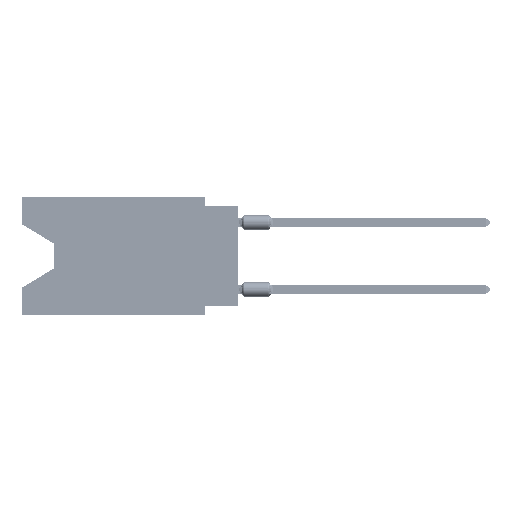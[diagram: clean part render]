
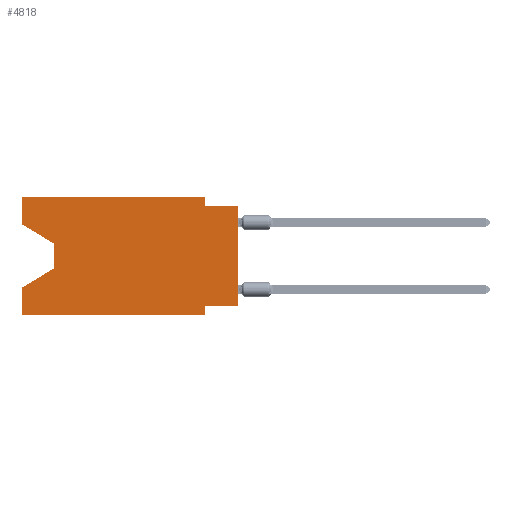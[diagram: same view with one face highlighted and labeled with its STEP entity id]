
A CAD part, left-side view. The second image highlights one B-rep face of the part: STEP entity #4818.
In plain terms, the highlighted planar face has unit normal (-1, 0, 0).
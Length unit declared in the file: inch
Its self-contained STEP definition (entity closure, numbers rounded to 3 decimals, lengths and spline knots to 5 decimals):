
#1222 = DIRECTION ( 'NONE',  ( 1., 0., 0. ) ) ;
#3884 = VERTEX_POINT ( 'NONE', #79119 ) ;
#4818 = ADVANCED_FACE ( 'NONE', ( #48601 ), #41045, .F. ) ;
#5077 = CARTESIAN_POINT ( 'NONE',  ( 0., 0.1, -0.35 ) ) ;
#6990 = VECTOR ( 'NONE', #43015, 39.37008 ) ;
#8329 = DIRECTION ( 'NONE',  ( 0., 0., -1. ) ) ;
#11922 = VERTEX_POINT ( 'NONE', #38605 ) ;
#16854 = DIRECTION ( 'NONE',  ( 0., 0., -1. ) ) ;
#16881 = VERTEX_POINT ( 'NONE', #51182 ) ;
#18978 = ORIENTED_EDGE ( 'NONE', *, *, #21117, .T. ) ;
#19656 = VERTEX_POINT ( 'NONE', #95528 ) ;
#19881 = VERTEX_POINT ( 'NONE', #33614 ) ;
#19899 = EDGE_CURVE ( 'NONE', #19881, #81661, #68547, .T. ) ;
#21117 = EDGE_CURVE ( 'NONE', #92996, #19881, #44362, .T. ) ;
#22657 = CARTESIAN_POINT ( 'NONE',  ( 0., 0.1, -0.35 ) ) ;
#23414 = CARTESIAN_POINT ( 'NONE',  ( 0., 0.645, -0.35 ) ) ;
#23574 = CARTESIAN_POINT ( 'NONE',  ( 0., 0.645, 0. ) ) ;
#24090 = LINE ( 'NONE', #23574, #85095 ) ;
#24146 = CARTESIAN_POINT ( 'NONE',  ( 0., 0.1, -0.325 ) ) ;
#24910 = CARTESIAN_POINT ( 'NONE',  ( 0., 0.645, 0. ) ) ;
#29621 = VECTOR ( 'NONE', #73208, 39.37008 ) ;
#30368 = VERTEX_POINT ( 'NONE', #24146 ) ;
#30608 = CARTESIAN_POINT ( 'NONE',  ( 0., 0.1, -0.025 ) ) ;
#31564 = ORIENTED_EDGE ( 'NONE', *, *, #97087, .F. ) ;
#31740 = DIRECTION ( 'NONE',  ( 0., 0., 1. ) ) ;
#33614 = CARTESIAN_POINT ( 'NONE',  ( 0., 0.55, -0.212 ) ) ;
#35190 = DIRECTION ( 'NONE',  ( 0., 0.855, -0.519 ) ) ;
#36057 = EDGE_CURVE ( 'NONE', #19656, #81661, #96804, .T. ) ;
#37345 = AXIS2_PLACEMENT_3D ( 'NONE', #24910, #1222, #16854 ) ;
#38605 = CARTESIAN_POINT ( 'NONE',  ( 0., 0., -0.325 ) ) ;
#40043 = DIRECTION ( 'NONE',  ( 0., -1., 0. ) ) ;
#40207 = DIRECTION ( 'NONE',  ( 0., -1., 0. ) ) ;
#40370 = VECTOR ( 'NONE', #35190, 39.37008 ) ;
#40494 = VERTEX_POINT ( 'NONE', #30608 ) ;
#41045 = PLANE ( 'NONE',  #37345 ) ;
#41357 = EDGE_CURVE ( 'NONE', #68279, #92996, #42521, .T. ) ;
#41616 = CARTESIAN_POINT ( 'NONE',  ( 0., 0., -0.025 ) ) ;
#42521 = LINE ( 'NONE', #44108, #58834 ) ;
#43015 = DIRECTION ( 'NONE',  ( 0., 0., 1. ) ) ;
#43273 = DIRECTION ( 'NONE',  ( 0., 0., -1. ) ) ;
#44108 = CARTESIAN_POINT ( 'NONE',  ( 0., 0.645, -0.08025 ) ) ;
#44270 = VECTOR ( 'NONE', #8329, 39.37008 ) ;
#44362 = LINE ( 'NONE', #84162, #79816 ) ;
#44863 = CARTESIAN_POINT ( 'NONE',  ( 0., 0., -0.325 ) ) ;
#46813 = DIRECTION ( 'NONE',  ( 0., 0., 1. ) ) ;
#48164 = LINE ( 'NONE', #23414, #97895 ) ;
#48601 = FACE_OUTER_BOUND ( 'NONE', #73057, .T. ) ;
#51182 = CARTESIAN_POINT ( 'NONE',  ( 0., 0.645, 0. ) ) ;
#54017 = VECTOR ( 'NONE', #46813, 39.37008 ) ;
#55703 = VERTEX_POINT ( 'NONE', #90023 ) ;
#56781 = CARTESIAN_POINT ( 'NONE',  ( 0., 0.1, 0. ) ) ;
#57452 = VECTOR ( 'NONE', #31740, 39.37008 ) ;
#58602 = CARTESIAN_POINT ( 'NONE',  ( 0., 0.645, -0.26975 ) ) ;
#58669 = EDGE_CURVE ( 'NONE', #3884, #40494, #97630, .T. ) ;
#58834 = VECTOR ( 'NONE', #83388, 39.37008 ) ;
#63979 = EDGE_CURVE ( 'NONE', #68279, #16881, #99487, .T. ) ;
#64314 = ORIENTED_EDGE ( 'NONE', *, *, #36057, .F. ) ;
#65839 = EDGE_CURVE ( 'NONE', #19656, #106133, #48164, .T. ) ;
#68013 = LINE ( 'NONE', #44863, #103574 ) ;
#68279 = VERTEX_POINT ( 'NONE', #96718 ) ;
#68547 = LINE ( 'NONE', #92220, #40370 ) ;
#69017 = EDGE_CURVE ( 'NONE', #30368, #106133, #87753, .T. ) ;
#72394 = ORIENTED_EDGE ( 'NONE', *, *, #41357, .T. ) ;
#73057 = EDGE_LOOP ( 'NONE', ( #72394, #18978, #102175, #64314, #76232, #89630, #31564, #76602, #97245, #106064, #102196, #100102 ) ) ;
#73208 = DIRECTION ( 'NONE',  ( 0., 0., -1. ) ) ;
#76232 = ORIENTED_EDGE ( 'NONE', *, *, #65839, .T. ) ;
#76602 = ORIENTED_EDGE ( 'NONE', *, *, #97984, .T. ) ;
#79074 = LINE ( 'NONE', #87699, #54017 ) ;
#79119 = CARTESIAN_POINT ( 'NONE',  ( 0., 0.1, 0. ) ) ;
#79816 = VECTOR ( 'NONE', #43273, 39.37008 ) ;
#80149 = CARTESIAN_POINT ( 'NONE',  ( 0., 0.645, 0. ) ) ;
#80244 = VECTOR ( 'NONE', #100202, 39.37008 ) ;
#81661 = VERTEX_POINT ( 'NONE', #58602 ) ;
#83388 = DIRECTION ( 'NONE',  ( 0., -0.855, -0.519 ) ) ;
#84162 = CARTESIAN_POINT ( 'NONE',  ( 0., 0.55, -0.138 ) ) ;
#85095 = VECTOR ( 'NONE', #40207, 39.37008 ) ;
#85206 = DIRECTION ( 'NONE',  ( 0., 1., 0. ) ) ;
#85486 = CARTESIAN_POINT ( 'NONE',  ( 0., 0.645, 0. ) ) ;
#87699 = CARTESIAN_POINT ( 'NONE',  ( 0., 0., 0. ) ) ;
#87753 = LINE ( 'NONE', #22657, #29621 ) ;
#89630 = ORIENTED_EDGE ( 'NONE', *, *, #69017, .F. ) ;
#90023 = CARTESIAN_POINT ( 'NONE',  ( 0., 0., -0.025 ) ) ;
#92220 = CARTESIAN_POINT ( 'NONE',  ( 0., 0.55, -0.212 ) ) ;
#92996 = VERTEX_POINT ( 'NONE', #104229 ) ;
#95528 = CARTESIAN_POINT ( 'NONE',  ( 0., 0.645, -0.35 ) ) ;
#96718 = CARTESIAN_POINT ( 'NONE',  ( 0., 0.645, -0.08025 ) ) ;
#96804 = LINE ( 'NONE', #80149, #57452 ) ;
#97087 = EDGE_CURVE ( 'NONE', #11922, #30368, #68013, .T. ) ;
#97245 = ORIENTED_EDGE ( 'NONE', *, *, #103068, .F. ) ;
#97630 = LINE ( 'NONE', #56781, #44270 ) ;
#97895 = VECTOR ( 'NONE', #40043, 39.37008 ) ;
#97984 = EDGE_CURVE ( 'NONE', #11922, #55703, #79074, .T. ) ;
#98629 = LINE ( 'NONE', #41616, #80244 ) ;
#99487 = LINE ( 'NONE', #85486, #6990 ) ;
#99703 = EDGE_CURVE ( 'NONE', #16881, #3884, #24090, .T. ) ;
#100102 = ORIENTED_EDGE ( 'NONE', *, *, #63979, .F. ) ;
#100202 = DIRECTION ( 'NONE',  ( 0., -1., 0. ) ) ;
#102175 = ORIENTED_EDGE ( 'NONE', *, *, #19899, .T. ) ;
#102196 = ORIENTED_EDGE ( 'NONE', *, *, #99703, .F. ) ;
#103068 = EDGE_CURVE ( 'NONE', #40494, #55703, #98629, .T. ) ;
#103574 = VECTOR ( 'NONE', #85206, 39.37008 ) ;
#104229 = CARTESIAN_POINT ( 'NONE',  ( 0., 0.55, -0.138 ) ) ;
#106064 = ORIENTED_EDGE ( 'NONE', *, *, #58669, .F. ) ;
#106133 = VERTEX_POINT ( 'NONE', #5077 ) ;
